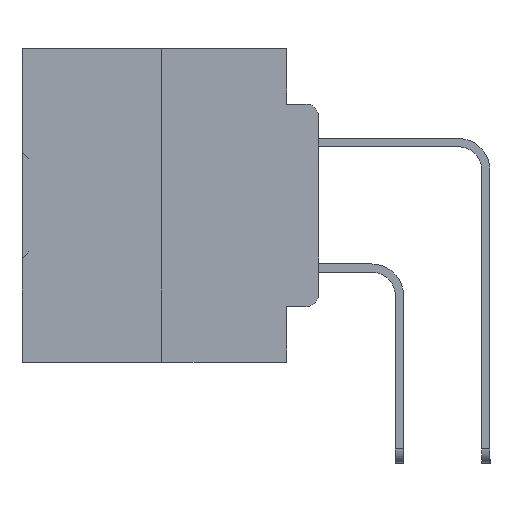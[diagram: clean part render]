
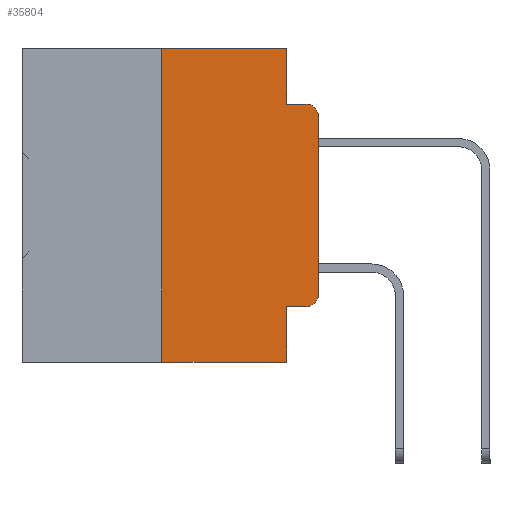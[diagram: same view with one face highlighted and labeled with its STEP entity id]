
A CAD part, left-side view. The second image highlights one B-rep face of the part: STEP entity #35804.
In plain terms, the highlighted planar face has unit normal (-1, 0, 0).
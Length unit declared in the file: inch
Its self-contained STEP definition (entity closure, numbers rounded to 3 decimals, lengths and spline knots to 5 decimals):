
#713 = CIRCLE ( 'NONE', #37247, 0.02 ) ;
#1636 = VERTEX_POINT ( 'NONE', #13006 ) ;
#2804 = VERTEX_POINT ( 'NONE', #41095 ) ;
#4276 = EDGE_CURVE ( 'NONE', #20863, #13714, #713, .T. ) ;
#4316 = CARTESIAN_POINT ( 'NONE',  ( 0., 0.25, 0. ) ) ;
#4430 = LINE ( 'NONE', #34474, #28752 ) ;
#4885 = DIRECTION ( 'NONE',  ( 0., -1., 0. ) ) ;
#7128 = DIRECTION ( 'NONE',  ( 0., 0., -1. ) ) ;
#7517 = VERTEX_POINT ( 'NONE', #18383 ) ;
#7635 = VECTOR ( 'NONE', #13905, 39.37008 ) ;
#8085 = LINE ( 'NONE', #36683, #15489 ) ;
#8104 = ORIENTED_EDGE ( 'NONE', *, *, #12096, .F. ) ;
#8800 = DIRECTION ( 'NONE',  ( 0., 0., 1. ) ) ;
#9246 = EDGE_CURVE ( 'NONE', #2804, #20863, #24178, .T. ) ;
#10847 = VECTOR ( 'NONE', #4885, 39.37008 ) ;
#11040 = CARTESIAN_POINT ( 'NONE',  ( 0., 0.051, -0.5 ) ) ;
#11041 = CARTESIAN_POINT ( 'NONE',  ( 0., 0.051, -0.4115 ) ) ;
#11177 = FACE_OUTER_BOUND ( 'NONE', #14725, .T. ) ;
#11710 = LINE ( 'NONE', #24612, #20159 ) ;
#11923 = EDGE_CURVE ( 'NONE', #34657, #7517, #34473, .T. ) ;
#11953 = CARTESIAN_POINT ( 'NONE',  ( 0., 0., -0.1085 ) ) ;
#12096 = EDGE_CURVE ( 'NONE', #2804, #18936, #22096, .T. ) ;
#12441 = LINE ( 'NONE', #34530, #19878 ) ;
#13006 = CARTESIAN_POINT ( 'NONE',  ( 0., 0.051, -0.0885 ) ) ;
#13042 = ORIENTED_EDGE ( 'NONE', *, *, #38958, .F. ) ;
#13714 = VERTEX_POINT ( 'NONE', #38367 ) ;
#13905 = DIRECTION ( 'NONE',  ( 0., -1., 0. ) ) ;
#14213 = DIRECTION ( 'NONE',  ( 0., -1., 0. ) ) ;
#14556 = DIRECTION ( 'NONE',  ( -1., 0., 0. ) ) ;
#14725 = EDGE_LOOP ( 'NONE', ( #18813, #17424, #13042, #31275, #28366, #35333, #23702, #8104, #36831, #17193 ) ) ;
#14766 = EDGE_CURVE ( 'NONE', #13714, #34657, #12441, .T. ) ;
#15489 = VECTOR ( 'NONE', #30336, 39.37008 ) ;
#16987 = CARTESIAN_POINT ( 'NONE',  ( 0., 0.02, -0.1085 ) ) ;
#17193 = ORIENTED_EDGE ( 'NONE', *, *, #4276, .T. ) ;
#17424 = ORIENTED_EDGE ( 'NONE', *, *, #11923, .T. ) ;
#18277 = LINE ( 'NONE', #23885, #10847 ) ;
#18383 = CARTESIAN_POINT ( 'NONE',  ( 0., 0.02, -0.0885 ) ) ;
#18813 = ORIENTED_EDGE ( 'NONE', *, *, #14766, .T. ) ;
#18936 = VERTEX_POINT ( 'NONE', #11040 ) ;
#19746 = PLANE ( 'NONE',  #23289 ) ;
#19878 = VECTOR ( 'NONE', #28180, 39.37008 ) ;
#20159 = VECTOR ( 'NONE', #8800, 39.37008 ) ;
#20209 = DIRECTION ( 'NONE',  ( 0., 0., -1. ) ) ;
#20344 = CARTESIAN_POINT ( 'NONE',  ( 0., 0.02, -0.4115 ) ) ;
#20863 = VERTEX_POINT ( 'NONE', #20344 ) ;
#22096 = LINE ( 'NONE', #39739, #29514 ) ;
#22186 = VERTEX_POINT ( 'NONE', #32613 ) ;
#22656 = AXIS2_PLACEMENT_3D ( 'NONE', #16987, #39193, #20209 ) ;
#22924 = CARTESIAN_POINT ( 'NONE',  ( 0., 0.473, 0. ) ) ;
#23289 = AXIS2_PLACEMENT_3D ( 'NONE', #22924, #35514, #7128 ) ;
#23702 = ORIENTED_EDGE ( 'NONE', *, *, #33159, .T. ) ;
#23885 = CARTESIAN_POINT ( 'NONE',  ( 0., 0.473, -0.5 ) ) ;
#24178 = LINE ( 'NONE', #11041, #40045 ) ;
#24612 = CARTESIAN_POINT ( 'NONE',  ( 0., 0.25, 0. ) ) ;
#26601 = VERTEX_POINT ( 'NONE', #38163 ) ;
#27132 = EDGE_CURVE ( 'NONE', #32252, #26601, #4430, .T. ) ;
#28180 = DIRECTION ( 'NONE',  ( 0., 0., 1. ) ) ;
#28366 = ORIENTED_EDGE ( 'NONE', *, *, #27132, .F. ) ;
#28752 = VECTOR ( 'NONE', #37695, 39.37008 ) ;
#29514 = VECTOR ( 'NONE', #36528, 39.37008 ) ;
#30336 = DIRECTION ( 'NONE',  ( 0., 0., -1. ) ) ;
#31275 = ORIENTED_EDGE ( 'NONE', *, *, #40346, .F. ) ;
#31941 = LINE ( 'NONE', #36089, #7635 ) ;
#32252 = VERTEX_POINT ( 'NONE', #4316 ) ;
#32613 = CARTESIAN_POINT ( 'NONE',  ( 0., 0.25, -0.5 ) ) ;
#33159 = EDGE_CURVE ( 'NONE', #22186, #18936, #18277, .T. ) ;
#33559 = CARTESIAN_POINT ( 'NONE',  ( 0., 0.02, -0.3915 ) ) ;
#34473 = CIRCLE ( 'NONE', #22656, 0.02 ) ;
#34474 = CARTESIAN_POINT ( 'NONE',  ( 0., 0.473, 0. ) ) ;
#34530 = CARTESIAN_POINT ( 'NONE',  ( 0., 0., 0. ) ) ;
#34657 = VERTEX_POINT ( 'NONE', #11953 ) ;
#35333 = ORIENTED_EDGE ( 'NONE', *, *, #37475, .F. ) ;
#35514 = DIRECTION ( 'NONE',  ( 1., 0., 0. ) ) ;
#35804 = ADVANCED_FACE ( 'NONE', ( #11177 ), #19746, .F. ) ;
#36089 = CARTESIAN_POINT ( 'NONE',  ( 0., 0.051, -0.0885 ) ) ;
#36528 = DIRECTION ( 'NONE',  ( 0., 0., -1. ) ) ;
#36683 = CARTESIAN_POINT ( 'NONE',  ( 0., 0.051, 0. ) ) ;
#36739 = DIRECTION ( 'NONE',  ( 0., 0., -1. ) ) ;
#36831 = ORIENTED_EDGE ( 'NONE', *, *, #9246, .T. ) ;
#37247 = AXIS2_PLACEMENT_3D ( 'NONE', #33559, #14556, #36739 ) ;
#37475 = EDGE_CURVE ( 'NONE', #22186, #32252, #11710, .T. ) ;
#37695 = DIRECTION ( 'NONE',  ( 0., -1., 0. ) ) ;
#38163 = CARTESIAN_POINT ( 'NONE',  ( 0., 0.051, 0. ) ) ;
#38367 = CARTESIAN_POINT ( 'NONE',  ( 0., 0., -0.3915 ) ) ;
#38958 = EDGE_CURVE ( 'NONE', #1636, #7517, #31941, .T. ) ;
#39193 = DIRECTION ( 'NONE',  ( -1., 0., 0. ) ) ;
#39739 = CARTESIAN_POINT ( 'NONE',  ( 0., 0.051, 0. ) ) ;
#40045 = VECTOR ( 'NONE', #14213, 39.37008 ) ;
#40346 = EDGE_CURVE ( 'NONE', #26601, #1636, #8085, .T. ) ;
#41095 = CARTESIAN_POINT ( 'NONE',  ( 0., 0.051, -0.4115 ) ) ;
